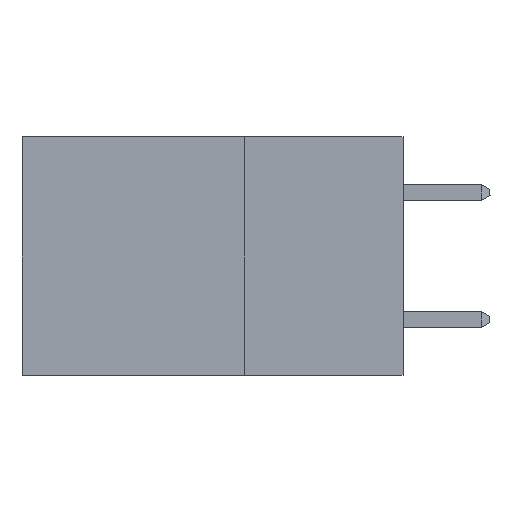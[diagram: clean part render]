
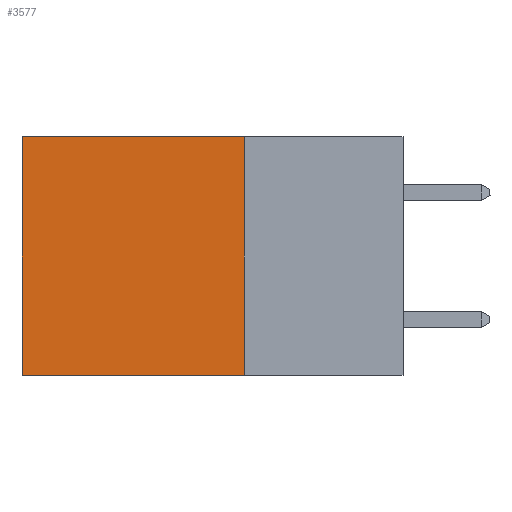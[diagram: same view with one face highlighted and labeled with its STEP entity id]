
A CAD part, left-side view. The second image highlights one B-rep face of the part: STEP entity #3577.
In plain terms, the highlighted planar face has unit normal (-1, 0, 0).
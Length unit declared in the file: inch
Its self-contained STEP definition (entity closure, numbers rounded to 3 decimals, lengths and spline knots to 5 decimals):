
#79 = LINE ( 'NONE', #2779, #6889 ) ;
#90 = CARTESIAN_POINT ( 'NONE',  ( 0.2875, 0.25, -0.375 ) ) ;
#423 = DIRECTION ( 'NONE',  ( 0., 1., 0. ) ) ;
#698 = DIRECTION ( 'NONE',  ( 1., 0., 0. ) ) ;
#910 = CARTESIAN_POINT ( 'NONE',  ( 0.2875, 0.6, 0. ) ) ;
#1150 = LINE ( 'NONE', #90, #1863 ) ;
#1222 = FACE_OUTER_BOUND ( 'NONE', #6370, .T. ) ;
#1411 = PLANE ( 'NONE',  #6893 ) ;
#1415 = DIRECTION ( 'NONE',  ( 0., 0., -1. ) ) ;
#1595 = ORIENTED_EDGE ( 'NONE', *, *, #3529, .T. ) ;
#1836 = CARTESIAN_POINT ( 'NONE',  ( 0.2875, 0.25, 0. ) ) ;
#1863 = VECTOR ( 'NONE', #1415, 39.37008 ) ;
#2506 = EDGE_CURVE ( 'NONE', #6011, #5509, #1150, .T. ) ;
#2579 = VERTEX_POINT ( 'NONE', #6753 ) ;
#2639 = LINE ( 'NONE', #1836, #3891 ) ;
#2779 = CARTESIAN_POINT ( 'NONE',  ( 0.2875, 0.6, -0.375 ) ) ;
#3092 = CARTESIAN_POINT ( 'NONE',  ( 0.2875, 0.25, -0.375 ) ) ;
#3508 = ORIENTED_EDGE ( 'NONE', *, *, #7632, .T. ) ;
#3529 = EDGE_CURVE ( 'NONE', #4262, #2579, #79, .T. ) ;
#3577 = ADVANCED_FACE ( 'NONE', ( #1222 ), #1411, .F. ) ;
#3625 = ORIENTED_EDGE ( 'NONE', *, *, #3919, .F. ) ;
#3891 = VECTOR ( 'NONE', #423, 39.37008 ) ;
#3919 = EDGE_CURVE ( 'NONE', #5509, #2579, #3995, .T. ) ;
#3995 = LINE ( 'NONE', #3092, #6770 ) ;
#4262 = VERTEX_POINT ( 'NONE', #910 ) ;
#4708 = DIRECTION ( 'NONE',  ( 0., 0., -1. ) ) ;
#4778 = CARTESIAN_POINT ( 'NONE',  ( 0.2875, 0.25, -0.375 ) ) ;
#5230 = CARTESIAN_POINT ( 'NONE',  ( 0.2875, 0.25, 0. ) ) ;
#5333 = DIRECTION ( 'NONE',  ( 0., 0., -1. ) ) ;
#5509 = VERTEX_POINT ( 'NONE', #4778 ) ;
#5826 = DIRECTION ( 'NONE',  ( 0., 1., 0. ) ) ;
#6011 = VERTEX_POINT ( 'NONE', #5230 ) ;
#6370 = EDGE_LOOP ( 'NONE', ( #1595, #3625, #7100, #3508 ) ) ;
#6753 = CARTESIAN_POINT ( 'NONE',  ( 0.2875, 0.6, -0.375 ) ) ;
#6770 = VECTOR ( 'NONE', #5826, 39.37008 ) ;
#6889 = VECTOR ( 'NONE', #5333, 39.37008 ) ;
#6893 = AXIS2_PLACEMENT_3D ( 'NONE', #7263, #698, #4708 ) ;
#7100 = ORIENTED_EDGE ( 'NONE', *, *, #2506, .F. ) ;
#7263 = CARTESIAN_POINT ( 'NONE',  ( 0.2875, 0.25, -0.375 ) ) ;
#7632 = EDGE_CURVE ( 'NONE', #6011, #4262, #2639, .T. ) ;
